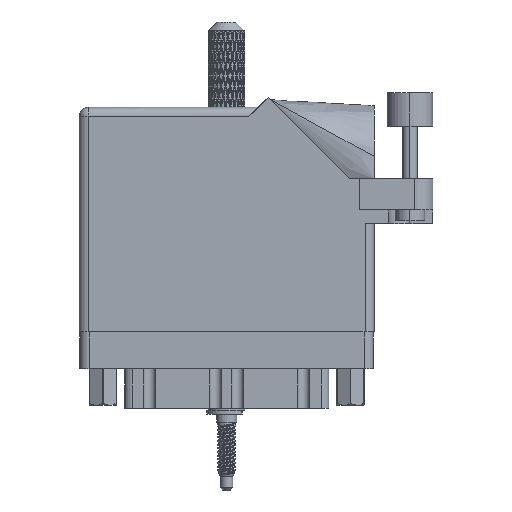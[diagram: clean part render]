
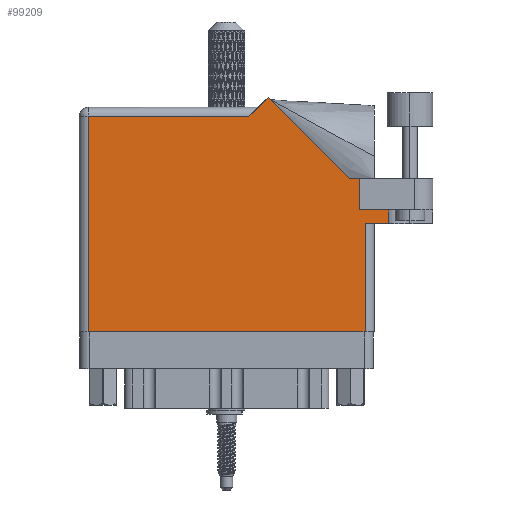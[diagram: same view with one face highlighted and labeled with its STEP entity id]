
A CAD part, front view. The second image highlights one B-rep face of the part: STEP entity #99209.
In plain terms, the highlighted face is planar.
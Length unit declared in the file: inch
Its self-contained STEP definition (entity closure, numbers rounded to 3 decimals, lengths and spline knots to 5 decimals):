
#2480 = LINE ( 'NONE', #55281, #105466 ) ;
#5773 = PLANE ( 'NONE',  #38844 ) ;
#5973 = LINE ( 'NONE', #23749, #10168 ) ;
#6342 = LINE ( 'NONE', #68835, #108709 ) ;
#6771 = EDGE_CURVE ( 'NONE', #40563, #29431, #8563, .T. ) ;
#8563 = LINE ( 'NONE', #69359, #88994 ) ;
#10168 = VECTOR ( 'NONE', #86264, 39.37008 ) ;
#12290 = CARTESIAN_POINT ( 'NONE',  ( 0., 1.53, 0. ) ) ;
#15022 = CARTESIAN_POINT ( 'NONE',  ( 1.948, 0.737, 0. ) ) ;
#15688 = VECTOR ( 'NONE', #35502, 39.37008 ) ;
#16115 = DIRECTION ( 'NONE',  ( -1., 0., 0. ) ) ;
#17951 = CARTESIAN_POINT ( 'NONE',  ( 1.91, 0.831, 0. ) ) ;
#20392 = CARTESIAN_POINT ( 'NONE',  ( 1.948, 0., 0. ) ) ;
#20674 = EDGE_CURVE ( 'NONE', #29431, #36212, #56489, .T. ) ;
#21488 = DIRECTION ( 'NONE',  ( 0., 1., 0. ) ) ;
#23254 = ORIENTED_EDGE ( 'NONE', *, *, #111165, .T. ) ;
#23643 = CARTESIAN_POINT ( 'NONE',  ( 2.1115, 0.737, 0. ) ) ;
#23749 = CARTESIAN_POINT ( 'NONE',  ( 1.84442, 1.044, 0. ) ) ;
#25783 = LINE ( 'NONE', #86043, #15688 ) ;
#28146 = ORIENTED_EDGE ( 'NONE', *, *, #60044, .T. ) ;
#29431 = VERTEX_POINT ( 'NONE', #20392 ) ;
#31830 = VECTOR ( 'NONE', #33456, 39.37008 ) ;
#32369 = VERTEX_POINT ( 'NONE', #59160 ) ;
#33423 = CARTESIAN_POINT ( 'NONE',  ( 1.91, 1.044, 0. ) ) ;
#33456 = DIRECTION ( 'NONE',  ( 1., 0., 0. ) ) ;
#33555 = CARTESIAN_POINT ( 'NONE',  ( 1.91, 0.831, 0. ) ) ;
#34000 = DIRECTION ( 'NONE',  ( 1., 0., 0. ) ) ;
#35502 = DIRECTION ( 'NONE',  ( 0., 1., 0. ) ) ;
#36212 = VERTEX_POINT ( 'NONE', #79925 ) ;
#36731 = DIRECTION ( 'NONE',  ( -1., 0., 0. ) ) ;
#37293 = LINE ( 'NONE', #106240, #87364 ) ;
#38844 = AXIS2_PLACEMENT_3D ( 'NONE', #12290, #41357, #16115 ) ;
#40563 = VERTEX_POINT ( 'NONE', #95658 ) ;
#40774 = CARTESIAN_POINT ( 'NONE',  ( 0.062, 0., 0. ) ) ;
#41349 = DIRECTION ( 'NONE',  ( 0., -1., 0. ) ) ;
#41357 = DIRECTION ( 'NONE',  ( 0., 0., -1. ) ) ;
#41950 = EDGE_CURVE ( 'NONE', #102017, #51063, #2480, .T. ) ;
#42361 = EDGE_CURVE ( 'NONE', #62318, #40563, #88446, .T. ) ;
#45969 = EDGE_CURVE ( 'NONE', #32369, #75844, #6342, .T. ) ;
#46046 = ORIENTED_EDGE ( 'NONE', *, *, #42361, .T. ) ;
#51063 = VERTEX_POINT ( 'NONE', #69538 ) ;
#51602 = DIRECTION ( 'NONE',  ( 1., 0., 0. ) ) ;
#55281 = CARTESIAN_POINT ( 'NONE',  ( 2.41, 1.044, 0. ) ) ;
#55944 = CARTESIAN_POINT ( 'NONE',  ( 1.217, 1.53, 0. ) ) ;
#56489 = LINE ( 'NONE', #15022, #93501 ) ;
#56575 = EDGE_CURVE ( 'NONE', #66116, #62318, #37293, .T. ) ;
#58183 = CARTESIAN_POINT ( 'NONE',  ( 2.01, 0.737, 0. ) ) ;
#59160 = CARTESIAN_POINT ( 'NONE',  ( 2.1115, 0.831, 0. ) ) ;
#60044 = EDGE_CURVE ( 'NONE', #86401, #102017, #25783, .T. ) ;
#61448 = ORIENTED_EDGE ( 'NONE', *, *, #72376, .T. ) ;
#62041 = EDGE_LOOP ( 'NONE', ( #91864, #96190, #81141, #72601, #84965, #28146, #107038, #23254, #61448, #83959, #46046 ) ) ;
#62318 = VERTEX_POINT ( 'NONE', #84431 ) ;
#63708 = VERTEX_POINT ( 'NONE', #106668 ) ;
#64444 = DIRECTION ( 'NONE',  ( -1., 0., 0. ) ) ;
#66116 = VERTEX_POINT ( 'NONE', #76816 ) ;
#66579 = DIRECTION ( 'NONE',  ( 0., -1., 0. ) ) ;
#68835 = CARTESIAN_POINT ( 'NONE',  ( 2.1115, 1.16177, 0. ) ) ;
#69359 = CARTESIAN_POINT ( 'NONE',  ( 0., 0., 0. ) ) ;
#69538 = CARTESIAN_POINT ( 'NONE',  ( 1.84442, 1.044, 0. ) ) ;
#69786 = VECTOR ( 'NONE', #34000, 39.37008 ) ;
#72376 = EDGE_CURVE ( 'NONE', #63708, #66116, #83445, .T. ) ;
#72601 = ORIENTED_EDGE ( 'NONE', *, *, #45969, .F. ) ;
#74340 = EDGE_CURVE ( 'NONE', #86401, #32369, #105763, .T. ) ;
#75844 = VERTEX_POINT ( 'NONE', #23643 ) ;
#76816 = CARTESIAN_POINT ( 'NONE',  ( 1.155, 1.468, 0. ) ) ;
#79925 = CARTESIAN_POINT ( 'NONE',  ( 1.948, 0.737, 0. ) ) ;
#81141 = ORIENTED_EDGE ( 'NONE', *, *, #87969, .T. ) ;
#82451 = VECTOR ( 'NONE', #109388, 39.37008 ) ;
#83445 = LINE ( 'NONE', #55944, #82451 ) ;
#83959 = ORIENTED_EDGE ( 'NONE', *, *, #56575, .T. ) ;
#84431 = CARTESIAN_POINT ( 'NONE',  ( 0.062, 1.468, 0. ) ) ;
#84921 = FACE_OUTER_BOUND ( 'NONE', #62041, .T. ) ;
#84965 = ORIENTED_EDGE ( 'NONE', *, *, #74340, .F. ) ;
#86043 = CARTESIAN_POINT ( 'NONE',  ( 1.91, 0.831, 0. ) ) ;
#86264 = DIRECTION ( 'NONE',  ( -0.707, 0.707, 0. ) ) ;
#86401 = VERTEX_POINT ( 'NONE', #33555 ) ;
#87364 = VECTOR ( 'NONE', #36731, 39.37008 ) ;
#87969 = EDGE_CURVE ( 'NONE', #36212, #75844, #94316, .T. ) ;
#88446 = LINE ( 'NONE', #40774, #94458 ) ;
#88994 = VECTOR ( 'NONE', #51602, 39.37008 ) ;
#91864 = ORIENTED_EDGE ( 'NONE', *, *, #6771, .T. ) ;
#93501 = VECTOR ( 'NONE', #21488, 39.37008 ) ;
#94316 = LINE ( 'NONE', #58183, #31830 ) ;
#94458 = VECTOR ( 'NONE', #66579, 39.37008 ) ;
#95658 = CARTESIAN_POINT ( 'NONE',  ( 0.062, 0., 0. ) ) ;
#96190 = ORIENTED_EDGE ( 'NONE', *, *, #20674, .T. ) ;
#99209 = ADVANCED_FACE ( 'NONE', ( #84921 ), #5773, .F. ) ;
#102017 = VERTEX_POINT ( 'NONE', #33423 ) ;
#105466 = VECTOR ( 'NONE', #64444, 39.37008 ) ;
#105763 = LINE ( 'NONE', #17951, #69786 ) ;
#106240 = CARTESIAN_POINT ( 'NONE',  ( 0., 1.468, 0. ) ) ;
#106668 = CARTESIAN_POINT ( 'NONE',  ( 1.28771, 1.60071, 0. ) ) ;
#107038 = ORIENTED_EDGE ( 'NONE', *, *, #41950, .T. ) ;
#108709 = VECTOR ( 'NONE', #41349, 39.37008 ) ;
#109388 = DIRECTION ( 'NONE',  ( -0.707, -0.707, 0. ) ) ;
#111165 = EDGE_CURVE ( 'NONE', #51063, #63708, #5973, .T. ) ;
